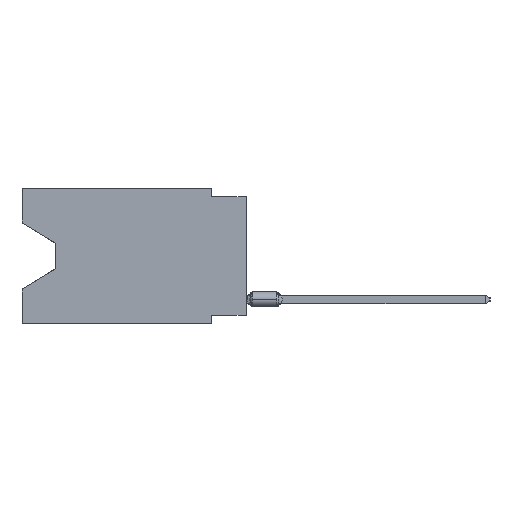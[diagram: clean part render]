
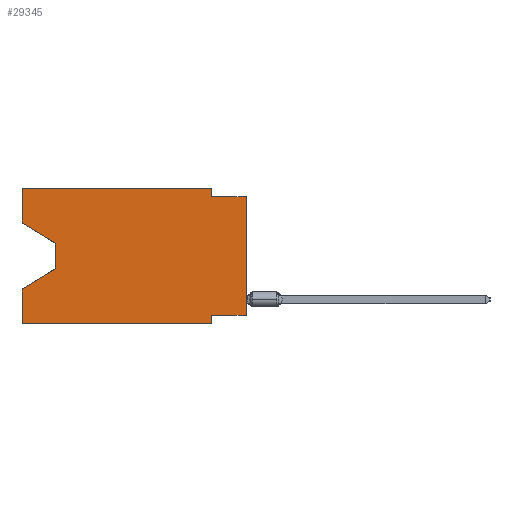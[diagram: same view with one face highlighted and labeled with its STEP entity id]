
A CAD part, left-side view. The second image highlights one B-rep face of the part: STEP entity #29345.
In plain terms, the highlighted planar face has unit normal (-1, 0, 0).
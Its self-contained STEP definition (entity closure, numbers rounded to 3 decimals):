
#611 = VERTEX_POINT ( 'NONE', #22036 ) ;
#612 = ORIENTED_EDGE ( 'NONE', *, *, #36076, .F. ) ;
#2206 = VECTOR ( 'NONE', #12478, 1000. ) ;
#2590 = VERTEX_POINT ( 'NONE', #28690 ) ;
#2658 = VERTEX_POINT ( 'NONE', #40090 ) ;
#2836 = CARTESIAN_POINT ( 'NONE',  ( 0., 0., -0.635 ) ) ;
#3066 = VECTOR ( 'NONE', #23877, 1000. ) ;
#3707 = EDGE_CURVE ( 'NONE', #2590, #24561, #8284, .T. ) ;
#3762 = CARTESIAN_POINT ( 'NONE',  ( 0., 16.383, 0. ) ) ;
#4637 = CARTESIAN_POINT ( 'NONE',  ( 0., 2.54, -9.906 ) ) ;
#4971 = VECTOR ( 'NONE', #41101, 1000. ) ;
#5226 = CARTESIAN_POINT ( 'NONE',  ( 0., 16.383, -9.906 ) ) ;
#5644 = LINE ( 'NONE', #14426, #4971 ) ;
#6150 = DIRECTION ( 'NONE',  ( 0., 0., -1. ) ) ;
#6517 = CARTESIAN_POINT ( 'NONE',  ( 0., 13.97, -4.013 ) ) ;
#6652 = VECTOR ( 'NONE', #23851, 1000. ) ;
#7208 = ORIENTED_EDGE ( 'NONE', *, *, #3707, .T. ) ;
#7509 = VERTEX_POINT ( 'NONE', #11156 ) ;
#8284 = LINE ( 'NONE', #23054, #9171 ) ;
#8514 = ORIENTED_EDGE ( 'NONE', *, *, #9994, .F. ) ;
#8534 = CARTESIAN_POINT ( 'NONE',  ( 0., 16.383, -7.36 ) ) ;
#8556 = VERTEX_POINT ( 'NONE', #4637 ) ;
#8912 = CARTESIAN_POINT ( 'NONE',  ( 0., 2.54, 0. ) ) ;
#9171 = VECTOR ( 'NONE', #46844, 1000. ) ;
#9304 = EDGE_CURVE ( 'NONE', #7509, #39321, #16870, .T. ) ;
#9388 = ORIENTED_EDGE ( 'NONE', *, *, #13871, .F. ) ;
#9994 = EDGE_CURVE ( 'NONE', #14701, #23395, #34779, .T. ) ;
#10266 = ORIENTED_EDGE ( 'NONE', *, *, #20146, .T. ) ;
#10467 = VECTOR ( 'NONE', #42687, 1000. ) ;
#11067 = VERTEX_POINT ( 'NONE', #8534 ) ;
#11156 = CARTESIAN_POINT ( 'NONE',  ( 0., 0., -9.271 ) ) ;
#11473 = CARTESIAN_POINT ( 'NONE',  ( 0., 16.383, 0. ) ) ;
#12478 = DIRECTION ( 'NONE',  ( 0., 0., 1. ) ) ;
#13753 = EDGE_CURVE ( 'NONE', #24561, #2658, #37590, .T. ) ;
#13871 = EDGE_CURVE ( 'NONE', #23395, #29762, #24170, .T. ) ;
#14426 = CARTESIAN_POINT ( 'NONE',  ( 0., 0., -9.271 ) ) ;
#14701 = VERTEX_POINT ( 'NONE', #50538 ) ;
#14928 = VECTOR ( 'NONE', #38913, 1000. ) ;
#15958 = ORIENTED_EDGE ( 'NONE', *, *, #40093, .F. ) ;
#16870 = LINE ( 'NONE', #31886, #2206 ) ;
#17115 = LINE ( 'NONE', #43518, #6652 ) ;
#19542 = DIRECTION ( 'NONE',  ( 1., 0., 0. ) ) ;
#19780 = PLANE ( 'NONE',  #51092 ) ;
#20146 = EDGE_CURVE ( 'NONE', #29918, #8556, #40520, .T. ) ;
#20197 = CARTESIAN_POINT ( 'NONE',  ( 0., 0., -0.635 ) ) ;
#21721 = CARTESIAN_POINT ( 'NONE',  ( 0., 2.54, 0. ) ) ;
#21874 = ORIENTED_EDGE ( 'NONE', *, *, #49920, .F. ) ;
#22036 = CARTESIAN_POINT ( 'NONE',  ( 0., 2.54, -9.271 ) ) ;
#22920 = FACE_OUTER_BOUND ( 'NONE', #34000, .T. ) ;
#23054 = CARTESIAN_POINT ( 'NONE',  ( 0., 16.383, -2.546 ) ) ;
#23395 = VERTEX_POINT ( 'NONE', #21721 ) ;
#23851 = DIRECTION ( 'NONE',  ( 0., 0.855, -0.519 ) ) ;
#23877 = DIRECTION ( 'NONE',  ( 0., 0., 1. ) ) ;
#24133 = VECTOR ( 'NONE', #33185, 1000. ) ;
#24170 = LINE ( 'NONE', #8912, #24958 ) ;
#24536 = VECTOR ( 'NONE', #30995, 1000. ) ;
#24561 = VERTEX_POINT ( 'NONE', #48626 ) ;
#24721 = DIRECTION ( 'NONE',  ( 0., -1., 0. ) ) ;
#24958 = VECTOR ( 'NONE', #35834, 1000. ) ;
#26327 = CARTESIAN_POINT ( 'NONE',  ( 0., 2.54, -9.906 ) ) ;
#27500 = CARTESIAN_POINT ( 'NONE',  ( 0., 2.54, -0.635 ) ) ;
#28690 = CARTESIAN_POINT ( 'NONE',  ( 0., 16.383, -2.546 ) ) ;
#29345 = ADVANCED_FACE ( 'NONE', ( #22920 ), #19780, .F. ) ;
#29762 = VERTEX_POINT ( 'NONE', #27500 ) ;
#29918 = VERTEX_POINT ( 'NONE', #5226 ) ;
#29944 = EDGE_CURVE ( 'NONE', #2658, #11067, #17115, .T. ) ;
#30741 = CARTESIAN_POINT ( 'NONE',  ( 0., 16.383, 0. ) ) ;
#30910 = CARTESIAN_POINT ( 'NONE',  ( 0., 16.383, 0. ) ) ;
#30995 = DIRECTION ( 'NONE',  ( 0., 0., 1. ) ) ;
#31886 = CARTESIAN_POINT ( 'NONE',  ( 0., 0., 0. ) ) ;
#31896 = LINE ( 'NONE', #30910, #3066 ) ;
#32618 = ORIENTED_EDGE ( 'NONE', *, *, #13753, .T. ) ;
#33185 = DIRECTION ( 'NONE',  ( 0., 0., -1. ) ) ;
#34000 = EDGE_LOOP ( 'NONE', ( #7208, #32618, #37779, #612, #10266, #37921, #21874, #47187, #42891, #9388, #8514, #15958 ) ) ;
#34405 = LINE ( 'NONE', #2836, #10467 ) ;
#34779 = LINE ( 'NONE', #11473, #14928 ) ;
#35583 = DIRECTION ( 'NONE',  ( 0., 0., -1. ) ) ;
#35658 = EDGE_CURVE ( 'NONE', #29762, #39321, #34405, .T. ) ;
#35834 = DIRECTION ( 'NONE',  ( 0., 0., -1. ) ) ;
#36076 = EDGE_CURVE ( 'NONE', #29918, #11067, #31896, .T. ) ;
#36651 = CARTESIAN_POINT ( 'NONE',  ( 0., 16.383, -9.906 ) ) ;
#37590 = LINE ( 'NONE', #6517, #24133 ) ;
#37779 = ORIENTED_EDGE ( 'NONE', *, *, #29944, .T. ) ;
#37921 = ORIENTED_EDGE ( 'NONE', *, *, #48691, .F. ) ;
#38913 = DIRECTION ( 'NONE',  ( 0., -1., 0. ) ) ;
#39321 = VERTEX_POINT ( 'NONE', #20197 ) ;
#40090 = CARTESIAN_POINT ( 'NONE',  ( 0., 13.97, -5.893 ) ) ;
#40093 = EDGE_CURVE ( 'NONE', #2590, #14701, #50891, .T. ) ;
#40520 = LINE ( 'NONE', #36651, #47980 ) ;
#41101 = DIRECTION ( 'NONE',  ( 0., 1., 0. ) ) ;
#42687 = DIRECTION ( 'NONE',  ( 0., -1., 0. ) ) ;
#42891 = ORIENTED_EDGE ( 'NONE', *, *, #35658, .F. ) ;
#43518 = CARTESIAN_POINT ( 'NONE',  ( 0., 13.97, -5.893 ) ) ;
#46844 = DIRECTION ( 'NONE',  ( 0., -0.855, -0.519 ) ) ;
#47187 = ORIENTED_EDGE ( 'NONE', *, *, #9304, .T. ) ;
#47980 = VECTOR ( 'NONE', #24721, 1000. ) ;
#48626 = CARTESIAN_POINT ( 'NONE',  ( 0., 13.97, -4.013 ) ) ;
#48691 = EDGE_CURVE ( 'NONE', #611, #8556, #48826, .T. ) ;
#48826 = LINE ( 'NONE', #26327, #50283 ) ;
#49920 = EDGE_CURVE ( 'NONE', #7509, #611, #5644, .T. ) ;
#50283 = VECTOR ( 'NONE', #6150, 1000. ) ;
#50538 = CARTESIAN_POINT ( 'NONE',  ( 0., 16.383, 0. ) ) ;
#50891 = LINE ( 'NONE', #30741, #24536 ) ;
#51092 = AXIS2_PLACEMENT_3D ( 'NONE', #3762, #19542, #35583 ) ;
